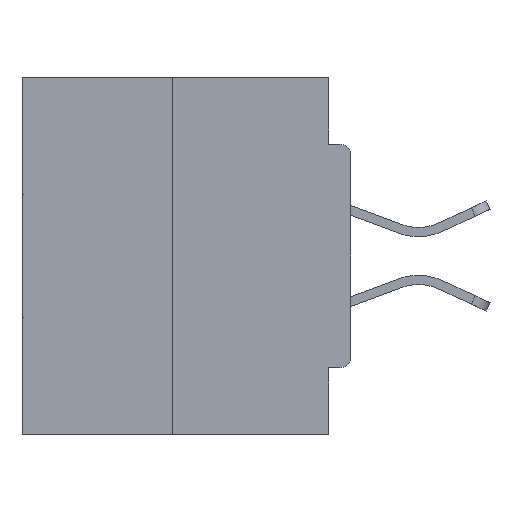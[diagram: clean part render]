
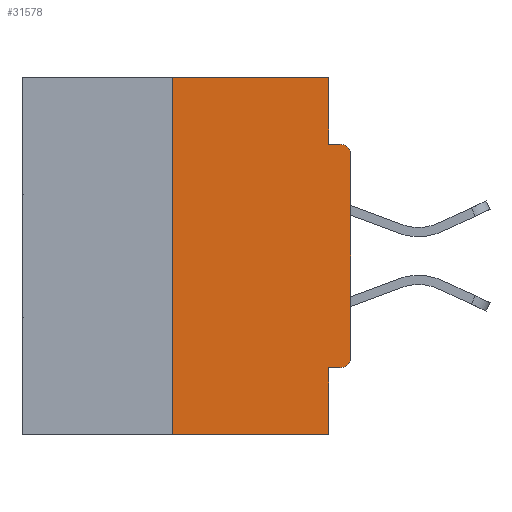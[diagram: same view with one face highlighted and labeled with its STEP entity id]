
A CAD part, left-side view. The second image highlights one B-rep face of the part: STEP entity #31578.
In plain terms, the highlighted planar face has unit normal (-1, 0, 0).
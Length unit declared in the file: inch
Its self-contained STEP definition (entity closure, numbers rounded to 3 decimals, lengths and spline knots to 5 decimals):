
#842 = ORIENTED_EDGE ( 'NONE', *, *, #14412, .F. ) ;
#1091 = VECTOR ( 'NONE', #36136, 39.37008 ) ;
#1378 = DIRECTION ( 'NONE',  ( -1., 0., 0. ) ) ;
#2024 = CARTESIAN_POINT ( 'NONE',  ( 0., 0.46, 0. ) ) ;
#2741 = ORIENTED_EDGE ( 'NONE', *, *, #28730, .F. ) ;
#3528 = AXIS2_PLACEMENT_3D ( 'NONE', #9603, #35433, #30087 ) ;
#4359 = DIRECTION ( 'NONE',  ( 0., 0., -1. ) ) ;
#5430 = CARTESIAN_POINT ( 'NONE',  ( 0., 0.031, 0. ) ) ;
#5738 = ORIENTED_EDGE ( 'NONE', *, *, #23220, .T. ) ;
#6407 = EDGE_LOOP ( 'NONE', ( #18427, #6946, #35700, #842, #2741, #22414, #12790, #5738, #13484, #10689 ) ) ;
#6836 = CIRCLE ( 'NONE', #30070, 0.015 ) ;
#6946 = ORIENTED_EDGE ( 'NONE', *, *, #25357, .F. ) ;
#8759 = DIRECTION ( 'NONE',  ( 0., 0., -1. ) ) ;
#9364 = DIRECTION ( 'NONE',  ( 0., 0., 1. ) ) ;
#9603 = CARTESIAN_POINT ( 'NONE',  ( 0., 0.015, -0.1085 ) ) ;
#10097 = VECTOR ( 'NONE', #8759, 39.37008 ) ;
#10122 = FACE_OUTER_BOUND ( 'NONE', #6407, .T. ) ;
#10152 = VERTEX_POINT ( 'NONE', #36226 ) ;
#10646 = VERTEX_POINT ( 'NONE', #12091 ) ;
#10689 = ORIENTED_EDGE ( 'NONE', *, *, #14139, .F. ) ;
#12091 = CARTESIAN_POINT ( 'NONE',  ( 0., 0.25, 0. ) ) ;
#12114 = LINE ( 'NONE', #32584, #34527 ) ;
#12790 = ORIENTED_EDGE ( 'NONE', *, *, #22103, .T. ) ;
#13092 = CARTESIAN_POINT ( 'NONE',  ( 0., 0.015, -0.3915 ) ) ;
#13484 = ORIENTED_EDGE ( 'NONE', *, *, #23465, .F. ) ;
#14139 = EDGE_CURVE ( 'NONE', #10152, #17093, #21552, .T. ) ;
#14412 = EDGE_CURVE ( 'NONE', #18507, #37971, #28355, .T. ) ;
#15086 = EDGE_CURVE ( 'NONE', #33263, #21018, #6836, .T. ) ;
#15457 = VERTEX_POINT ( 'NONE', #28179 ) ;
#15566 = VECTOR ( 'NONE', #33059, 39.37008 ) ;
#15656 = VECTOR ( 'NONE', #16858, 39.37008 ) ;
#16726 = CARTESIAN_POINT ( 'NONE',  ( 0., 0.25, 0. ) ) ;
#16858 = DIRECTION ( 'NONE',  ( 0., 0., 1. ) ) ;
#17093 = VERTEX_POINT ( 'NONE', #28077 ) ;
#18292 = CARTESIAN_POINT ( 'NONE',  ( 0., 0., 0. ) ) ;
#18427 = ORIENTED_EDGE ( 'NONE', *, *, #23030, .F. ) ;
#18469 = CARTESIAN_POINT ( 'NONE',  ( 0., 0., -0.4065 ) ) ;
#18480 = CIRCLE ( 'NONE', #3528, 0.015 ) ;
#18507 = VERTEX_POINT ( 'NONE', #33379 ) ;
#20739 = CARTESIAN_POINT ( 'NONE',  ( 0., 0.031, -0.5 ) ) ;
#21018 = VERTEX_POINT ( 'NONE', #32377 ) ;
#21091 = CARTESIAN_POINT ( 'NONE',  ( 0., 0.46, 0. ) ) ;
#21552 = LINE ( 'NONE', #5430, #10097 ) ;
#21853 = VECTOR ( 'NONE', #9364, 39.37008 ) ;
#21925 = CARTESIAN_POINT ( 'NONE',  ( 0., 0.015, -0.0935 ) ) ;
#22103 = EDGE_CURVE ( 'NONE', #21018, #26061, #35056, .T. ) ;
#22411 = PLANE ( 'NONE',  #23338 ) ;
#22414 = ORIENTED_EDGE ( 'NONE', *, *, #15086, .T. ) ;
#23030 = EDGE_CURVE ( 'NONE', #10646, #10152, #23108, .T. ) ;
#23108 = LINE ( 'NONE', #21091, #30446 ) ;
#23126 = LINE ( 'NONE', #18469, #1091 ) ;
#23184 = VERTEX_POINT ( 'NONE', #21925 ) ;
#23220 = EDGE_CURVE ( 'NONE', #26061, #23184, #18480, .T. ) ;
#23338 = AXIS2_PLACEMENT_3D ( 'NONE', #2024, #25602, #25359 ) ;
#23410 = LINE ( 'NONE', #16726, #15656 ) ;
#23465 = EDGE_CURVE ( 'NONE', #17093, #23184, #12114, .T. ) ;
#23583 = CARTESIAN_POINT ( 'NONE',  ( 0., 0.46, -0.5 ) ) ;
#23789 = VECTOR ( 'NONE', #29511, 39.37008 ) ;
#24466 = CARTESIAN_POINT ( 'NONE',  ( 0., 0.031, -0.5 ) ) ;
#25357 = EDGE_CURVE ( 'NONE', #15457, #10646, #23410, .T. ) ;
#25359 = DIRECTION ( 'NONE',  ( 0., 0., -1. ) ) ;
#25602 = DIRECTION ( 'NONE',  ( 1., 0., 0. ) ) ;
#26061 = VERTEX_POINT ( 'NONE', #27505 ) ;
#27505 = CARTESIAN_POINT ( 'NONE',  ( 0., 0., -0.1085 ) ) ;
#28077 = CARTESIAN_POINT ( 'NONE',  ( 0., 0.031, -0.0935 ) ) ;
#28179 = CARTESIAN_POINT ( 'NONE',  ( 0., 0.25, -0.5 ) ) ;
#28355 = LINE ( 'NONE', #24466, #15566 ) ;
#28730 = EDGE_CURVE ( 'NONE', #33263, #18507, #23126, .T. ) ;
#29511 = DIRECTION ( 'NONE',  ( 0., -1., 0. ) ) ;
#30070 = AXIS2_PLACEMENT_3D ( 'NONE', #13092, #1378, #4359 ) ;
#30087 = DIRECTION ( 'NONE',  ( 0., 0., -1. ) ) ;
#30446 = VECTOR ( 'NONE', #35638, 39.37008 ) ;
#31112 = LINE ( 'NONE', #23583, #23789 ) ;
#31543 = CARTESIAN_POINT ( 'NONE',  ( 0., 0.015, -0.4065 ) ) ;
#31578 = ADVANCED_FACE ( 'NONE', ( #10122 ), #22411, .F. ) ;
#32320 = EDGE_CURVE ( 'NONE', #15457, #37971, #31112, .T. ) ;
#32377 = CARTESIAN_POINT ( 'NONE',  ( 0., 0., -0.3915 ) ) ;
#32584 = CARTESIAN_POINT ( 'NONE',  ( 0., 0., -0.0935 ) ) ;
#32959 = DIRECTION ( 'NONE',  ( 0., -1., 0. ) ) ;
#33059 = DIRECTION ( 'NONE',  ( 0., 0., -1. ) ) ;
#33263 = VERTEX_POINT ( 'NONE', #31543 ) ;
#33379 = CARTESIAN_POINT ( 'NONE',  ( 0., 0.031, -0.4065 ) ) ;
#34527 = VECTOR ( 'NONE', #32959, 39.37008 ) ;
#35056 = LINE ( 'NONE', #18292, #21853 ) ;
#35433 = DIRECTION ( 'NONE',  ( -1., 0., 0. ) ) ;
#35638 = DIRECTION ( 'NONE',  ( 0., -1., 0. ) ) ;
#35700 = ORIENTED_EDGE ( 'NONE', *, *, #32320, .T. ) ;
#36136 = DIRECTION ( 'NONE',  ( 0., 1., 0. ) ) ;
#36226 = CARTESIAN_POINT ( 'NONE',  ( 0., 0.031, 0. ) ) ;
#37971 = VERTEX_POINT ( 'NONE', #20739 ) ;
